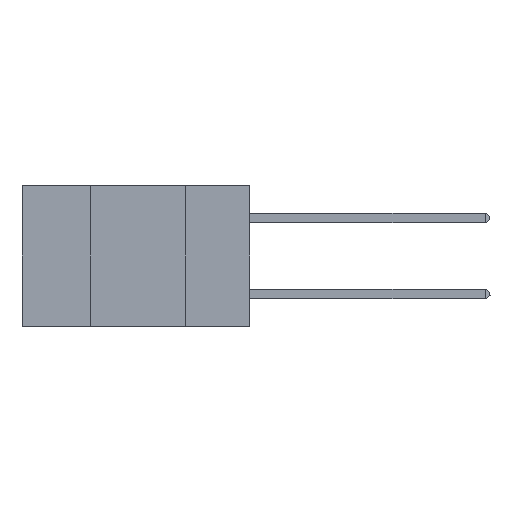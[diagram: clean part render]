
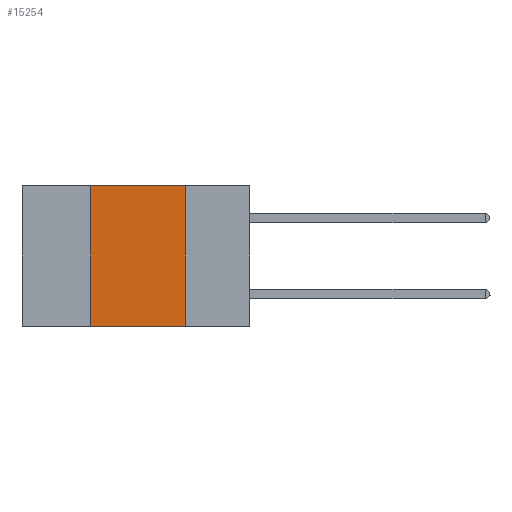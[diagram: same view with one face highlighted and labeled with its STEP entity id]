
A CAD part, left-side view. The second image highlights one B-rep face of the part: STEP entity #15254.
In plain terms, the highlighted planar face has unit normal (-1, 0, 0).
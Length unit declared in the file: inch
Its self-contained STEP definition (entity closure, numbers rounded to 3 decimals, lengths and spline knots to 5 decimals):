
#10 = LINE ( 'NONE', #6341, #28298 ) ;
#1143 = EDGE_CURVE ( 'NONE', #28845, #27053, #14425, .T. ) ;
#1295 = AXIS2_PLACEMENT_3D ( 'NONE', #3135, #13871, #8918 ) ;
#1761 = VERTEX_POINT ( 'NONE', #11151 ) ;
#3135 = CARTESIAN_POINT ( 'NONE',  ( 0., 0.6, 0. ) ) ;
#3650 = FACE_OUTER_BOUND ( 'NONE', #16764, .T. ) ;
#4732 = CARTESIAN_POINT ( 'NONE',  ( 0., 0.42, 0. ) ) ;
#5025 = CARTESIAN_POINT ( 'NONE',  ( 0., 0.17, 0. ) ) ;
#6086 = LINE ( 'NONE', #9348, #28813 ) ;
#6341 = CARTESIAN_POINT ( 'NONE',  ( 0., 0.42, 0. ) ) ;
#7036 = DIRECTION ( 'NONE',  ( 0., 0., -1. ) ) ;
#8918 = DIRECTION ( 'NONE',  ( 0., 0., -1. ) ) ;
#9348 = CARTESIAN_POINT ( 'NONE',  ( 0., 0.6, -0.37 ) ) ;
#11151 = CARTESIAN_POINT ( 'NONE',  ( 0., 0.42, -0.37 ) ) ;
#12111 = DIRECTION ( 'NONE',  ( 0., -1., 0. ) ) ;
#13871 = DIRECTION ( 'NONE',  ( 1., 0., 0. ) ) ;
#14153 = LINE ( 'NONE', #30737, #34796 ) ;
#14175 = ORIENTED_EDGE ( 'NONE', *, *, #30345, .F. ) ;
#14425 = LINE ( 'NONE', #15288, #19502 ) ;
#15254 = ADVANCED_FACE ( 'NONE', ( #3650 ), #21877, .F. ) ;
#15288 = CARTESIAN_POINT ( 'NONE',  ( 0., 0.17, 0. ) ) ;
#16764 = EDGE_LOOP ( 'NONE', ( #20086, #14175, #29243, #27440 ) ) ;
#19502 = VECTOR ( 'NONE', #7036, 39.37008 ) ;
#20086 = ORIENTED_EDGE ( 'NONE', *, *, #1143, .F. ) ;
#21877 = PLANE ( 'NONE',  #1295 ) ;
#27053 = VERTEX_POINT ( 'NONE', #27634 ) ;
#27440 = ORIENTED_EDGE ( 'NONE', *, *, #33670, .T. ) ;
#27634 = CARTESIAN_POINT ( 'NONE',  ( 0., 0.17, -0.37 ) ) ;
#28298 = VECTOR ( 'NONE', #29981, 39.37008 ) ;
#28813 = VECTOR ( 'NONE', #33166, 39.37008 ) ;
#28845 = VERTEX_POINT ( 'NONE', #5025 ) ;
#29243 = ORIENTED_EDGE ( 'NONE', *, *, #34842, .F. ) ;
#29981 = DIRECTION ( 'NONE',  ( 0., 0., 1. ) ) ;
#30345 = EDGE_CURVE ( 'NONE', #34009, #28845, #14153, .T. ) ;
#30737 = CARTESIAN_POINT ( 'NONE',  ( 0., 0.6, 0. ) ) ;
#33166 = DIRECTION ( 'NONE',  ( 0., -1., 0. ) ) ;
#33670 = EDGE_CURVE ( 'NONE', #1761, #27053, #6086, .T. ) ;
#34009 = VERTEX_POINT ( 'NONE', #4732 ) ;
#34796 = VECTOR ( 'NONE', #12111, 39.37008 ) ;
#34842 = EDGE_CURVE ( 'NONE', #1761, #34009, #10, .T. ) ;
